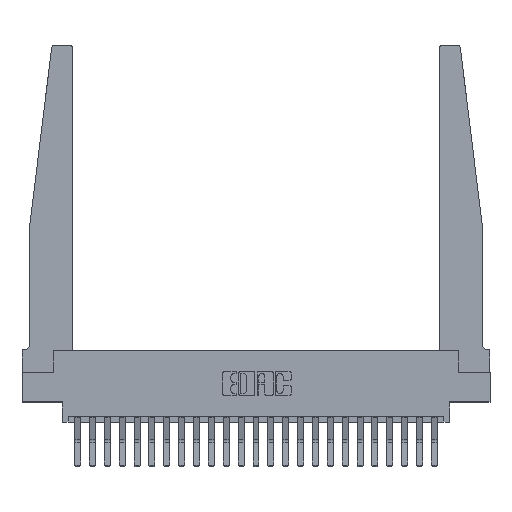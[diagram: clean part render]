
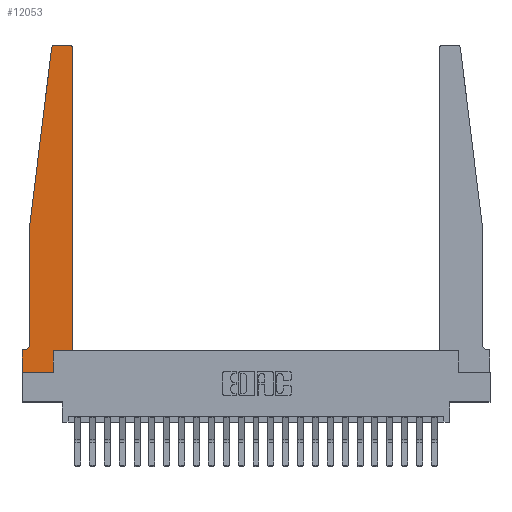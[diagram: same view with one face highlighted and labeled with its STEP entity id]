
A CAD part, top view. The second image highlights one B-rep face of the part: STEP entity #12053.
In plain terms, the highlighted planar face has unit normal (0, 0, 1).
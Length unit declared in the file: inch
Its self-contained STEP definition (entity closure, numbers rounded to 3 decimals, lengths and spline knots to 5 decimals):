
#220 = DIRECTION ( 'NONE',  ( 0., -1., 0. ) ) ;
#267 = EDGE_CURVE ( 'NONE', #16874, #1473, #18557, .T. ) ;
#525 = AXIS2_PLACEMENT_3D ( 'NONE', #7186, #19997, #9017 ) ;
#910 = EDGE_CURVE ( 'NONE', #22518, #21855, #10713, .T. ) ;
#938 = LINE ( 'NONE', #22532, #10031 ) ;
#1225 = VERTEX_POINT ( 'NONE', #15437 ) ;
#1473 = VERTEX_POINT ( 'NONE', #21636 ) ;
#1504 = EDGE_CURVE ( 'NONE', #8579, #14612, #9013, .T. ) ;
#1857 = ORIENTED_EDGE ( 'NONE', *, *, #6546, .T. ) ;
#2133 = ORIENTED_EDGE ( 'NONE', *, *, #910, .T. ) ;
#2261 = VECTOR ( 'NONE', #9007, 39.37008 ) ;
#2284 = LINE ( 'NONE', #12086, #8268 ) ;
#2722 = EDGE_CURVE ( 'NONE', #14612, #16874, #15808, .T. ) ;
#2991 = ORIENTED_EDGE ( 'NONE', *, *, #5150, .T. ) ;
#3553 = CARTESIAN_POINT ( 'NONE',  ( 0.425, 2.72, 0.37 ) ) ;
#3661 = CARTESIAN_POINT ( 'NONE',  ( 0.2605, 0., 0.37 ) ) ;
#3772 = VERTEX_POINT ( 'NONE', #19719 ) ;
#4213 = CARTESIAN_POINT ( 'NONE',  ( 0., 0.1875, 0.37 ) ) ;
#4328 = CARTESIAN_POINT ( 'NONE',  ( 0., 0.1875, 0.37 ) ) ;
#4380 = CARTESIAN_POINT ( 'NONE',  ( 0.065, 0.2375, 0.37 ) ) ;
#4747 = VERTEX_POINT ( 'NONE', #4328 ) ;
#5118 = EDGE_CURVE ( 'NONE', #20551, #3772, #16283, .T. ) ;
#5150 = EDGE_CURVE ( 'NONE', #1225, #12436, #10760, .T. ) ;
#5501 = DIRECTION ( 'NONE',  ( 0., 1., 0. ) ) ;
#5518 = CARTESIAN_POINT ( 'NONE',  ( 0.015, 0.2375, 0.37 ) ) ;
#5945 = DIRECTION ( 'NONE',  ( -1., 0., 0. ) ) ;
#5985 = DIRECTION ( 'NONE',  ( 0., 0., 1. ) ) ;
#6020 = DIRECTION ( 'NONE',  ( 1., 0., 0. ) ) ;
#6546 = EDGE_CURVE ( 'NONE', #12436, #8579, #18267, .T. ) ;
#6597 = DIRECTION ( 'NONE',  ( 0., -1., 0. ) ) ;
#7186 = CARTESIAN_POINT ( 'NONE',  ( 0.27653, 2.72, 0.37 ) ) ;
#7251 = CARTESIAN_POINT ( 'NONE',  ( 0.2605, 0.18, 0.37 ) ) ;
#7303 = VECTOR ( 'NONE', #16239, 39.37008 ) ;
#7355 = DIRECTION ( 'NONE',  ( -1., 0., 0. ) ) ;
#7510 = CARTESIAN_POINT ( 'NONE',  ( 0.015, 0.1875, 0.37 ) ) ;
#7644 = CARTESIAN_POINT ( 'NONE',  ( 0.395, 2.75, 0.37 ) ) ;
#8225 = VECTOR ( 'NONE', #8522, 39.37008 ) ;
#8268 = VECTOR ( 'NONE', #6597, 39.37008 ) ;
#8522 = DIRECTION ( 'NONE',  ( -0.122, -0.992, 0. ) ) ;
#8579 = VERTEX_POINT ( 'NONE', #7644 ) ;
#9007 = DIRECTION ( 'NONE',  ( 0., 1., 0. ) ) ;
#9013 = LINE ( 'NONE', #21712, #7303 ) ;
#9017 = DIRECTION ( 'NONE',  ( 1., 0., 0. ) ) ;
#9538 = ORIENTED_EDGE ( 'NONE', *, *, #5118, .T. ) ;
#9819 = EDGE_CURVE ( 'NONE', #4747, #13291, #2284, .T. ) ;
#10031 = VECTOR ( 'NONE', #17067, 39.37008 ) ;
#10713 = CIRCLE ( 'NONE', #13707, 0.05 ) ;
#10740 = EDGE_CURVE ( 'NONE', #13291, #20551, #13953, .T. ) ;
#10760 = LINE ( 'NONE', #10965, #11334 ) ;
#10965 = CARTESIAN_POINT ( 'NONE',  ( 0.425, 0.18, 0.37 ) ) ;
#11334 = VECTOR ( 'NONE', #5501, 39.37008 ) ;
#11475 = CARTESIAN_POINT ( 'NONE',  ( 0., 0., 0.37 ) ) ;
#12015 = EDGE_CURVE ( 'NONE', #21855, #4747, #18248, .T. ) ;
#12053 = ADVANCED_FACE ( 'NONE', ( #21352 ), #22407, .T. ) ;
#12086 = CARTESIAN_POINT ( 'NONE',  ( 0., 0., 0.37 ) ) ;
#12380 = ORIENTED_EDGE ( 'NONE', *, *, #14670, .T. ) ;
#12436 = VERTEX_POINT ( 'NONE', #3553 ) ;
#12757 = VECTOR ( 'NONE', #5945, 39.37008 ) ;
#12971 = ORIENTED_EDGE ( 'NONE', *, *, #267, .T. ) ;
#13270 = DIRECTION ( 'NONE',  ( 1., 0., 0. ) ) ;
#13291 = VERTEX_POINT ( 'NONE', #20385 ) ;
#13707 = AXIS2_PLACEMENT_3D ( 'NONE', #5518, #18345, #7355 ) ;
#13953 = LINE ( 'NONE', #11475, #14527 ) ;
#14095 = LINE ( 'NONE', #14817, #18968 ) ;
#14527 = VECTOR ( 'NONE', #13270, 39.37008 ) ;
#14612 = VERTEX_POINT ( 'NONE', #16519 ) ;
#14627 = AXIS2_PLACEMENT_3D ( 'NONE', #4213, #17023, #6020 ) ;
#14670 = EDGE_CURVE ( 'NONE', #1473, #22518, #14095, .T. ) ;
#14817 = CARTESIAN_POINT ( 'NONE',  ( 0.065, 1.25, 0.37 ) ) ;
#14848 = EDGE_CURVE ( 'NONE', #3772, #1225, #938, .T. ) ;
#15001 = ORIENTED_EDGE ( 'NONE', *, *, #9819, .T. ) ;
#15437 = CARTESIAN_POINT ( 'NONE',  ( 0.425, 0.18, 0.37 ) ) ;
#15808 = CIRCLE ( 'NONE', #525, 0.03 ) ;
#15988 = EDGE_LOOP ( 'NONE', ( #19017, #23258, #12971, #12380, #2133, #20995, #15001, #19314, #9538, #17607, #2991, #1857 ) ) ;
#16239 = DIRECTION ( 'NONE',  ( -1., 0., 0. ) ) ;
#16283 = LINE ( 'NONE', #7251, #2261 ) ;
#16519 = CARTESIAN_POINT ( 'NONE',  ( 0.27653, 2.75, 0.37 ) ) ;
#16532 = CARTESIAN_POINT ( 'NONE',  ( 0.24675, 2.72367, 0.37 ) ) ;
#16638 = CARTESIAN_POINT ( 'NONE',  ( 0.065, 1.25, 0.37 ) ) ;
#16874 = VERTEX_POINT ( 'NONE', #16532 ) ;
#16979 = CARTESIAN_POINT ( 'NONE',  ( 0.395, 2.72, 0.37 ) ) ;
#17023 = DIRECTION ( 'NONE',  ( 0., 0., 1. ) ) ;
#17067 = DIRECTION ( 'NONE',  ( 1., 0., 0. ) ) ;
#17607 = ORIENTED_EDGE ( 'NONE', *, *, #14848, .T. ) ;
#18248 = LINE ( 'NONE', #22325, #12757 ) ;
#18267 = CIRCLE ( 'NONE', #23104, 0.03 ) ;
#18345 = DIRECTION ( 'NONE',  ( 0., 0., -1. ) ) ;
#18557 = LINE ( 'NONE', #16638, #8225 ) ;
#18817 = DIRECTION ( 'NONE',  ( 1., 0., 0. ) ) ;
#18968 = VECTOR ( 'NONE', #220, 39.37008 ) ;
#19017 = ORIENTED_EDGE ( 'NONE', *, *, #1504, .T. ) ;
#19314 = ORIENTED_EDGE ( 'NONE', *, *, #10740, .T. ) ;
#19719 = CARTESIAN_POINT ( 'NONE',  ( 0.2605, 0.18, 0.37 ) ) ;
#19997 = DIRECTION ( 'NONE',  ( 0., 0., 1. ) ) ;
#20385 = CARTESIAN_POINT ( 'NONE',  ( 0., 0., 0.37 ) ) ;
#20551 = VERTEX_POINT ( 'NONE', #3661 ) ;
#20995 = ORIENTED_EDGE ( 'NONE', *, *, #12015, .T. ) ;
#21352 = FACE_OUTER_BOUND ( 'NONE', #15988, .T. ) ;
#21636 = CARTESIAN_POINT ( 'NONE',  ( 0.065, 1.25, 0.37 ) ) ;
#21712 = CARTESIAN_POINT ( 'NONE',  ( 0.25, 2.75, 0.37 ) ) ;
#21855 = VERTEX_POINT ( 'NONE', #7510 ) ;
#22325 = CARTESIAN_POINT ( 'NONE',  ( 0.065, 0.1875, 0.37 ) ) ;
#22407 = PLANE ( 'NONE',  #14627 ) ;
#22518 = VERTEX_POINT ( 'NONE', #4380 ) ;
#22532 = CARTESIAN_POINT ( 'NONE',  ( 0.425, 0.18, 0.37 ) ) ;
#23104 = AXIS2_PLACEMENT_3D ( 'NONE', #16979, #5985, #18817 ) ;
#23258 = ORIENTED_EDGE ( 'NONE', *, *, #2722, .T. ) ;
